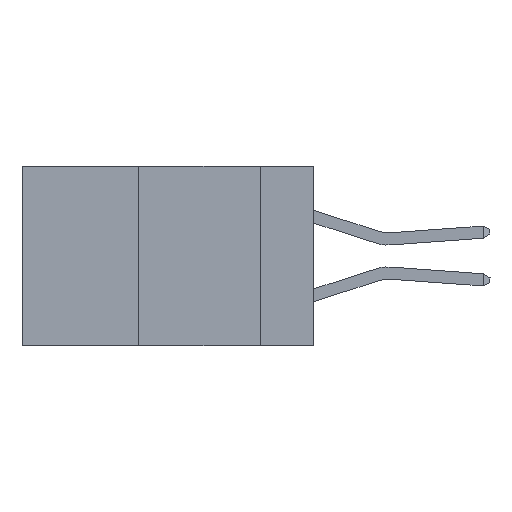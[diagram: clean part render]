
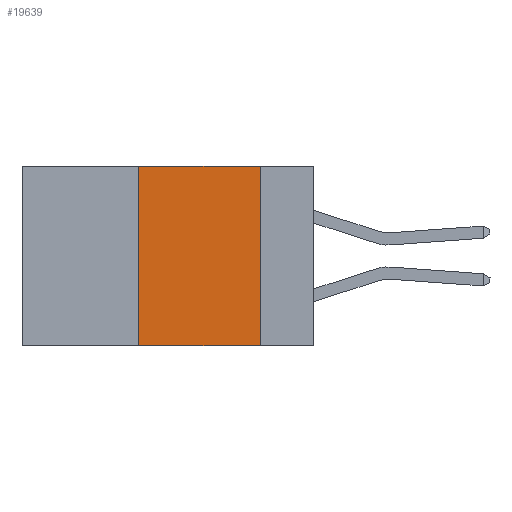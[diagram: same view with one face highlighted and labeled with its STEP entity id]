
A CAD part, left-side view. The second image highlights one B-rep face of the part: STEP entity #19639.
In plain terms, the highlighted planar face has unit normal (-1, 0, 0).
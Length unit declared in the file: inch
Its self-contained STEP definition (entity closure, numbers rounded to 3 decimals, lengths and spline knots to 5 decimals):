
#699 = LINE ( 'NONE', #17767, #21704 ) ;
#1311 = ORIENTED_EDGE ( 'NONE', *, *, #39310, .F. ) ;
#2949 = VECTOR ( 'NONE', #6595, 39.37008 ) ;
#3726 = VECTOR ( 'NONE', #31438, 39.37008 ) ;
#3994 = VERTEX_POINT ( 'NONE', #40648 ) ;
#4559 = CARTESIAN_POINT ( 'NONE',  ( 0., 0.36, 0. ) ) ;
#6365 = FACE_OUTER_BOUND ( 'NONE', #14153, .T. ) ;
#6595 = DIRECTION ( 'NONE',  ( 0., 0., 1. ) ) ;
#6904 = CARTESIAN_POINT ( 'NONE',  ( 0., 0.6, -0.37 ) ) ;
#9265 = VERTEX_POINT ( 'NONE', #4559 ) ;
#10275 = LINE ( 'NONE', #40358, #2949 ) ;
#10395 = EDGE_CURVE ( 'NONE', #9265, #24449, #699, .T. ) ;
#11347 = CARTESIAN_POINT ( 'NONE',  ( 0., 0.11, 0. ) ) ;
#11987 = LINE ( 'NONE', #11347, #3726 ) ;
#14153 = EDGE_LOOP ( 'NONE', ( #35057, #33798, #1311, #21525 ) ) ;
#14703 = VECTOR ( 'NONE', #26383, 39.37008 ) ;
#16323 = DIRECTION ( 'NONE',  ( 0., 0., -1. ) ) ;
#16548 = CARTESIAN_POINT ( 'NONE',  ( 0., 0.11, -0.37 ) ) ;
#16761 = PLANE ( 'NONE',  #34636 ) ;
#17141 = DIRECTION ( 'NONE',  ( 0., -1., 0. ) ) ;
#17767 = CARTESIAN_POINT ( 'NONE',  ( 0., 0.6, 0. ) ) ;
#19639 = ADVANCED_FACE ( 'NONE', ( #6365 ), #16761, .F. ) ;
#19743 = CARTESIAN_POINT ( 'NONE',  ( 0., 0.11, 0. ) ) ;
#21525 = ORIENTED_EDGE ( 'NONE', *, *, #31231, .T. ) ;
#21704 = VECTOR ( 'NONE', #17141, 39.37008 ) ;
#24449 = VERTEX_POINT ( 'NONE', #19743 ) ;
#26300 = VERTEX_POINT ( 'NONE', #16548 ) ;
#26383 = DIRECTION ( 'NONE',  ( 0., -1., 0. ) ) ;
#29089 = DIRECTION ( 'NONE',  ( 1., 0., 0. ) ) ;
#31231 = EDGE_CURVE ( 'NONE', #3994, #26300, #32267, .T. ) ;
#31438 = DIRECTION ( 'NONE',  ( 0., 0., -1. ) ) ;
#32267 = LINE ( 'NONE', #6904, #14703 ) ;
#33798 = ORIENTED_EDGE ( 'NONE', *, *, #10395, .F. ) ;
#34636 = AXIS2_PLACEMENT_3D ( 'NONE', #36217, #29089, #16323 ) ;
#35057 = ORIENTED_EDGE ( 'NONE', *, *, #40842, .F. ) ;
#36217 = CARTESIAN_POINT ( 'NONE',  ( 0., 0.6, 0. ) ) ;
#39310 = EDGE_CURVE ( 'NONE', #3994, #9265, #10275, .T. ) ;
#40358 = CARTESIAN_POINT ( 'NONE',  ( 0., 0.36, 0. ) ) ;
#40648 = CARTESIAN_POINT ( 'NONE',  ( 0., 0.36, -0.37 ) ) ;
#40842 = EDGE_CURVE ( 'NONE', #24449, #26300, #11987, .T. ) ;
